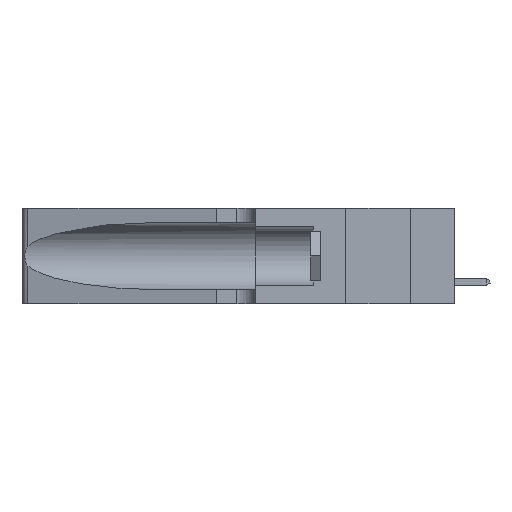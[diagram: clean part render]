
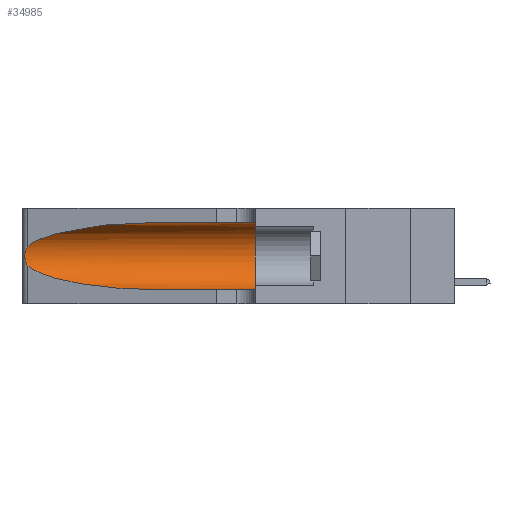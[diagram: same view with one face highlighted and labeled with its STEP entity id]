
A CAD part, left-side view. The second image highlights one B-rep face of the part: STEP entity #34985.
In plain terms, the highlighted cylindrical face has radius 3.308 mm (diameter 6.617 mm), a partial arc.
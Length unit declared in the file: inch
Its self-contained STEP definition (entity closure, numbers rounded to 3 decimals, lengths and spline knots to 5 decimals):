
#181 = CARTESIAN_POINT ( 'NONE',  ( 0.25487, 1.22718, 0.22369 ) ) ;
#306 = AXIS2_PLACEMENT_3D ( 'NONE', #36633, #36468, #12810 ) ;
#1044 = CARTESIAN_POINT ( 'NONE',  ( 0.26017, 1.23833, 0.17102 ) ) ;
#1425 = DIRECTION ( 'NONE',  ( 0., 0., 1. ) ) ;
#1797 = CARTESIAN_POINT ( 'NONE',  ( 0.1305, 0.72297, 0.31525 ) ) ;
#2373 = CYLINDRICAL_SURFACE ( 'NONE', #306, 0.13025 ) ;
#2407 = CARTESIAN_POINT ( 'NONE',  ( 0.1305, 0.35, 0.05475 ) ) ;
#4293 = EDGE_CURVE ( 'NONE', #48957, #10566, #21377, .T. ) ;
#4298 = ORIENTED_EDGE ( 'NONE', *, *, #5805, .T. ) ;
#4429 = ORIENTED_EDGE ( 'NONE', *, *, #25829, .T. ) ;
#4679 = VERTEX_POINT ( 'NONE', #1797 ) ;
#5478 = CARTESIAN_POINT ( 'NONE',  ( 0.2373, 1.15595, 0.28018 ) ) ;
#5805 = EDGE_CURVE ( 'NONE', #43938, #18105, #29135, .T. ) ;
#6767 = CARTESIAN_POINT ( 'NONE',  ( 0.25487, 1.22718, 0.22369 ) ) ;
#9276 = CARTESIAN_POINT ( 'NONE',  ( 0.25787, 1.23484, 0.2124 ) ) ;
#9897 = DIRECTION ( 'NONE',  ( 0., 1., 0. ) ) ;
#10335 = CARTESIAN_POINT ( 'NONE',  ( 0.1305, 0.35, 0.185 ) ) ;
#10566 = VERTEX_POINT ( 'NONE', #2407 ) ;
#11816 = CARTESIAN_POINT ( 'NONE',  ( 0.25555, 1.22994, 0.2215 ) ) ;
#12751 = CARTESIAN_POINT ( 'NONE',  ( 0.25854, 1.2359, 0.20912 ) ) ;
#12810 = DIRECTION ( 'NONE',  ( 0., 0., -1. ) ) ;
#12988 = ORIENTED_EDGE ( 'NONE', *, *, #49909, .T. ) ;
#13711 = VERTEX_POINT ( 'NONE', #14922 ) ;
#14068 = CARTESIAN_POINT ( 'NONE',  ( 0.25487, 1.22718, 0.14631 ) ) ;
#14608 = VECTOR ( 'NONE', #50551, 39.37008 ) ;
#14922 = CARTESIAN_POINT ( 'NONE',  ( 0.25487, 1.22718, 0.22369 ) ) ;
#16864 = CARTESIAN_POINT ( 'NONE',  ( 0.26075, 1.23896, 0.178 ) ) ;
#18105 = VERTEX_POINT ( 'NONE', #40290 ) ;
#18438 = CARTESIAN_POINT ( 'NONE',  ( 0.1305, 0.72297, 0.05475 ) ) ;
#18808 = CARTESIAN_POINT ( 'NONE',  ( 0.2373, 1.15595, 0.08982 ) ) ;
#19392 =( BOUNDED_CURVE ( )  B_SPLINE_CURVE ( 3, ( #41598, #29919, #5478, #6767 ),
 .UNSPECIFIED., .F., .T. ) 
 B_SPLINE_CURVE_WITH_KNOTS ( ( 4, 4 ),
 ( 1.5708, 2.84003 ),
 .UNSPECIFIED. ) 
 CURVE ( )  GEOMETRIC_REPRESENTATION_ITEM ( )  RATIONAL_B_SPLINE_CURVE ( ( 1., 0.87, 0.87, 1. ) ) 
 REPRESENTATION_ITEM ( '' )  );
#20371 = CARTESIAN_POINT ( 'NONE',  ( 0.25856, 1.23593, 0.16098 ) ) ;
#20527 = CARTESIAN_POINT ( 'NONE',  ( 0.25639, 1.23186, 0.15144 ) ) ;
#21032 = CARTESIAN_POINT ( 'NONE',  ( 0.25789, 1.23486, 0.15765 ) ) ;
#21374 = EDGE_LOOP ( 'NONE', ( #46188, #12988, #4298, #4429, #47026, #21832 ) ) ;
#21377 = CIRCLE ( 'NONE', #31721, 0.13025 ) ;
#21832 = ORIENTED_EDGE ( 'NONE', *, *, #26423, .F. ) ;
#24505 = CARTESIAN_POINT ( 'NONE',  ( 0.25555, 1.22993, 0.14849 ) ) ;
#24878 = DIRECTION ( 'NONE',  ( 0., -1., 0. ) ) ;
#25143 = VECTOR ( 'NONE', #24878, 39.37008 ) ;
#25829 = EDGE_CURVE ( 'NONE', #18105, #10566, #46929, .T. ) ;
#26423 = EDGE_CURVE ( 'NONE', #4679, #48957, #41070, .T. ) ;
#28650 = CARTESIAN_POINT ( 'NONE',  ( 0.26018, 1.23835, 0.19895 ) ) ;
#28822 = CARTESIAN_POINT ( 'NONE',  ( 0.25487, 1.22718, 0.14631 ) ) ;
#29135 =( BOUNDED_CURVE ( )  B_SPLINE_CURVE ( 3, ( #14068, #18808, #50049, #18438 ),
 .UNSPECIFIED., .F., .F. ) 
 B_SPLINE_CURVE_WITH_KNOTS ( ( 4, 4 ),
 ( 3.44316, 4.71239 ),
 .UNSPECIFIED. ) 
 CURVE ( )  GEOMETRIC_REPRESENTATION_ITEM ( )  RATIONAL_B_SPLINE_CURVE ( ( 1., 0.87, 0.87, 1. ) ) 
 REPRESENTATION_ITEM ( '' )  );
#29919 = CARTESIAN_POINT ( 'NONE',  ( 0.18966, 0.96281, 0.31525 ) ) ;
#30525 = CARTESIAN_POINT ( 'NONE',  ( 0.25487, 1.22718, 0.14631 ) ) ;
#31721 = AXIS2_PLACEMENT_3D ( 'NONE', #10335, #9897, #1425 ) ;
#34985 = ADVANCED_FACE ( 'NONE', ( #43245 ), #2373, .F. ) ;
#36468 = DIRECTION ( 'NONE',  ( 0., -1., 0. ) ) ;
#36633 = CARTESIAN_POINT ( 'NONE',  ( 0.1305, 1.61858, 0.185 ) ) ;
#39450 = CARTESIAN_POINT ( 'NONE',  ( 0.25639, 1.23184, 0.21858 ) ) ;
#40290 = CARTESIAN_POINT ( 'NONE',  ( 0.1305, 0.72297, 0.05475 ) ) ;
#41070 = LINE ( 'NONE', #42922, #14608 ) ;
#41598 = CARTESIAN_POINT ( 'NONE',  ( 0.1305, 0.72297, 0.31525 ) ) ;
#42922 = CARTESIAN_POINT ( 'NONE',  ( 0.1305, 1.61858, 0.31525 ) ) ;
#43245 = FACE_OUTER_BOUND ( 'NONE', #21374, .T. ) ;
#43938 = VERTEX_POINT ( 'NONE', #30525 ) ;
#44067 = CARTESIAN_POINT ( 'NONE',  ( 0.1305, 1.61858, 0.05475 ) ) ;
#46188 = ORIENTED_EDGE ( 'NONE', *, *, #50189, .T. ) ;
#46929 = LINE ( 'NONE', #44067, #25143 ) ;
#47026 = ORIENTED_EDGE ( 'NONE', *, *, #4293, .F. ) ;
#48035 = CARTESIAN_POINT ( 'NONE',  ( 0.26075, 1.23896, 0.19203 ) ) ;
#48830 = CARTESIAN_POINT ( 'NONE',  ( 0.1305, 0.35, 0.31525 ) ) ;
#48957 = VERTEX_POINT ( 'NONE', #48830 ) ;
#49909 = EDGE_CURVE ( 'NONE', #13711, #43938, #50751, .T. ) ;
#50049 = CARTESIAN_POINT ( 'NONE',  ( 0.18966, 0.96281, 0.05475 ) ) ;
#50189 = EDGE_CURVE ( 'NONE', #4679, #13711, #19392, .T. ) ;
#50551 = DIRECTION ( 'NONE',  ( 0., -1., 0. ) ) ;
#50751 = B_SPLINE_CURVE_WITH_KNOTS ( 'NONE', 3,
 ( #181, #11816, #39450, #9276, #12751, #28650, #48035, #16864, #1044, #20371, #21032, #20527, #24505, #28822 ),
 .UNSPECIFIED., .F., .F.,
 ( 4, 2, 2, 2, 2, 2, 4 ),
 ( 0., 0.00027, 0.00053, 0.00107, 0.0016, 0.00187, 0.00214 ),
 .UNSPECIFIED. ) ;
